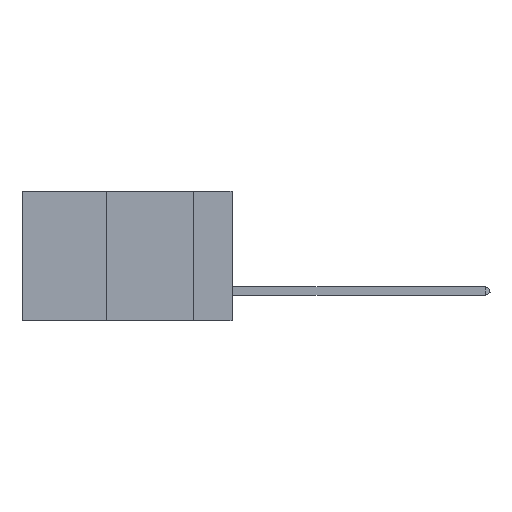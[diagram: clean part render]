
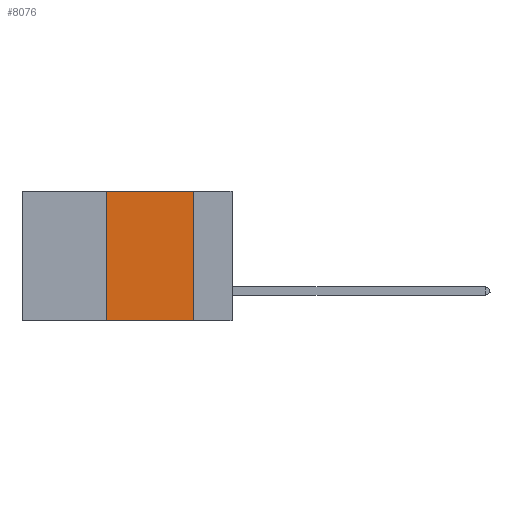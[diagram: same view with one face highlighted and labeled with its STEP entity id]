
A CAD part, left-side view. The second image highlights one B-rep face of the part: STEP entity #8076.
In plain terms, the highlighted planar face has unit normal (-1, 0, 0).
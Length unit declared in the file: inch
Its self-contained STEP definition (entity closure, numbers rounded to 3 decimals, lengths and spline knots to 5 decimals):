
#382 = EDGE_LOOP ( 'NONE', ( #3691, #8758, #6353, #1810 ) ) ;
#393 = DIRECTION ( 'NONE',  ( 0., -1., 0. ) ) ;
#407 = CARTESIAN_POINT ( 'NONE',  ( 0., 0.11, -0.37 ) ) ;
#815 = EDGE_CURVE ( 'NONE', #2653, #9430, #2621, .T. ) ;
#829 = DIRECTION ( 'NONE',  ( 0., 0., -1. ) ) ;
#962 = EDGE_CURVE ( 'NONE', #6789, #2653, #10113, .T. ) ;
#1558 = CARTESIAN_POINT ( 'NONE',  ( 0., 0.36, 0. ) ) ;
#1810 = ORIENTED_EDGE ( 'NONE', *, *, #8513, .T. ) ;
#1929 = CARTESIAN_POINT ( 'NONE',  ( 0., 0.36, 0. ) ) ;
#2621 = LINE ( 'NONE', #8052, #3318 ) ;
#2653 = VERTEX_POINT ( 'NONE', #1558 ) ;
#2733 = DIRECTION ( 'NONE',  ( 1., 0., 0. ) ) ;
#2768 = FACE_OUTER_BOUND ( 'NONE', #382, .T. ) ;
#3318 = VECTOR ( 'NONE', #8092, 39.37008 ) ;
#3691 = ORIENTED_EDGE ( 'NONE', *, *, #5139, .F. ) ;
#4510 = CARTESIAN_POINT ( 'NONE',  ( 0., 0.6, 0. ) ) ;
#4608 = DIRECTION ( 'NONE',  ( 0., 0., 1. ) ) ;
#5139 = EDGE_CURVE ( 'NONE', #9430, #6143, #7468, .T. ) ;
#5907 = VECTOR ( 'NONE', #4608, 39.37008 ) ;
#6143 = VERTEX_POINT ( 'NONE', #407 ) ;
#6177 = AXIS2_PLACEMENT_3D ( 'NONE', #4510, #2733, #829 ) ;
#6353 = ORIENTED_EDGE ( 'NONE', *, *, #962, .F. ) ;
#6789 = VERTEX_POINT ( 'NONE', #10941 ) ;
#7188 = PLANE ( 'NONE',  #6177 ) ;
#7299 = CARTESIAN_POINT ( 'NONE',  ( 0., 0.11, 0. ) ) ;
#7468 = LINE ( 'NONE', #8368, #8651 ) ;
#7502 = DIRECTION ( 'NONE',  ( 0., 0., -1. ) ) ;
#8052 = CARTESIAN_POINT ( 'NONE',  ( 0., 0.6, 0. ) ) ;
#8076 = ADVANCED_FACE ( 'NONE', ( #2768 ), #7188, .F. ) ;
#8092 = DIRECTION ( 'NONE',  ( 0., -1., 0. ) ) ;
#8368 = CARTESIAN_POINT ( 'NONE',  ( 0., 0.11, 0. ) ) ;
#8513 = EDGE_CURVE ( 'NONE', #6789, #6143, #8545, .T. ) ;
#8545 = LINE ( 'NONE', #8699, #11835 ) ;
#8651 = VECTOR ( 'NONE', #7502, 39.37008 ) ;
#8699 = CARTESIAN_POINT ( 'NONE',  ( 0., 0.6, -0.37 ) ) ;
#8758 = ORIENTED_EDGE ( 'NONE', *, *, #815, .F. ) ;
#9430 = VERTEX_POINT ( 'NONE', #7299 ) ;
#10113 = LINE ( 'NONE', #1929, #5907 ) ;
#10941 = CARTESIAN_POINT ( 'NONE',  ( 0., 0.36, -0.37 ) ) ;
#11835 = VECTOR ( 'NONE', #393, 39.37008 ) ;
